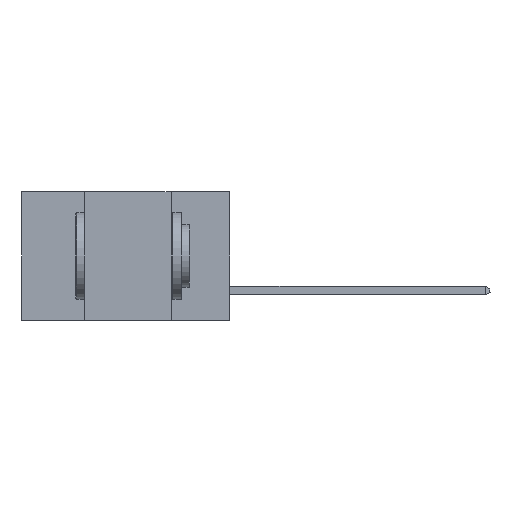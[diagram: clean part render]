
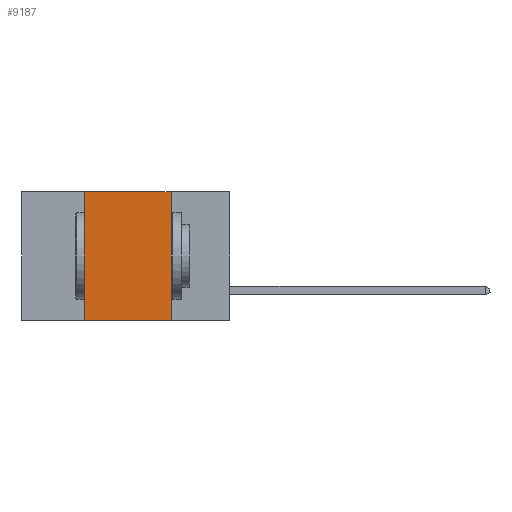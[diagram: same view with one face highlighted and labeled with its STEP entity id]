
A CAD part, left-side view. The second image highlights one B-rep face of the part: STEP entity #9187.
In plain terms, the highlighted planar face has unit normal (-1, 0, 0).
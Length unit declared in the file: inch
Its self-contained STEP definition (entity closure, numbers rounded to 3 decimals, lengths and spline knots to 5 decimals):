
#221 = ORIENTED_EDGE ( 'NONE', *, *, #5498, .F. ) ;
#756 = ORIENTED_EDGE ( 'NONE', *, *, #2499, .F. ) ;
#918 = CARTESIAN_POINT ( 'NONE',  ( 0., 0.6, 0. ) ) ;
#1377 = VECTOR ( 'NONE', #10252, 39.37008 ) ;
#1897 = PLANE ( 'NONE',  #4760 ) ;
#2499 = EDGE_CURVE ( 'NONE', #6728, #13970, #3534, .T. ) ;
#2795 = LINE ( 'NONE', #4535, #1377 ) ;
#2870 = DIRECTION ( 'NONE',  ( 0., 0., -1. ) ) ;
#3227 = ORIENTED_EDGE ( 'NONE', *, *, #5999, .T. ) ;
#3308 = LINE ( 'NONE', #10146, #7333 ) ;
#3528 = VERTEX_POINT ( 'NONE', #13699 ) ;
#3534 = LINE ( 'NONE', #918, #6489 ) ;
#3542 = VECTOR ( 'NONE', #2870, 39.37008 ) ;
#3580 = VERTEX_POINT ( 'NONE', #13803 ) ;
#4535 = CARTESIAN_POINT ( 'NONE',  ( 0., 0.6, -0.37 ) ) ;
#4760 = AXIS2_PLACEMENT_3D ( 'NONE', #10929, #5123, #11910 ) ;
#5123 = DIRECTION ( 'NONE',  ( 1., 0., 0. ) ) ;
#5498 = EDGE_CURVE ( 'NONE', #13970, #3580, #12340, .T. ) ;
#5914 = CARTESIAN_POINT ( 'NONE',  ( 0., 0.17, 0. ) ) ;
#5999 = EDGE_CURVE ( 'NONE', #3528, #3580, #2795, .T. ) ;
#6217 = EDGE_LOOP ( 'NONE', ( #221, #756, #10320, #3227 ) ) ;
#6489 = VECTOR ( 'NONE', #13357, 39.37008 ) ;
#6728 = VERTEX_POINT ( 'NONE', #11825 ) ;
#7061 = EDGE_CURVE ( 'NONE', #3528, #6728, #3308, .T. ) ;
#7333 = VECTOR ( 'NONE', #11171, 39.37008 ) ;
#9187 = ADVANCED_FACE ( 'NONE', ( #9606 ), #1897, .F. ) ;
#9606 = FACE_OUTER_BOUND ( 'NONE', #6217, .T. ) ;
#10146 = CARTESIAN_POINT ( 'NONE',  ( 0., 0.42, 0. ) ) ;
#10252 = DIRECTION ( 'NONE',  ( 0., -1., 0. ) ) ;
#10320 = ORIENTED_EDGE ( 'NONE', *, *, #7061, .F. ) ;
#10929 = CARTESIAN_POINT ( 'NONE',  ( 0., 0.6, 0. ) ) ;
#11171 = DIRECTION ( 'NONE',  ( 0., 0., 1. ) ) ;
#11825 = CARTESIAN_POINT ( 'NONE',  ( 0., 0.42, 0. ) ) ;
#11910 = DIRECTION ( 'NONE',  ( 0., 0., -1. ) ) ;
#11989 = CARTESIAN_POINT ( 'NONE',  ( 0., 0.17, 0. ) ) ;
#12340 = LINE ( 'NONE', #11989, #3542 ) ;
#13357 = DIRECTION ( 'NONE',  ( 0., -1., 0. ) ) ;
#13699 = CARTESIAN_POINT ( 'NONE',  ( 0., 0.42, -0.37 ) ) ;
#13803 = CARTESIAN_POINT ( 'NONE',  ( 0., 0.17, -0.37 ) ) ;
#13970 = VERTEX_POINT ( 'NONE', #5914 ) ;
